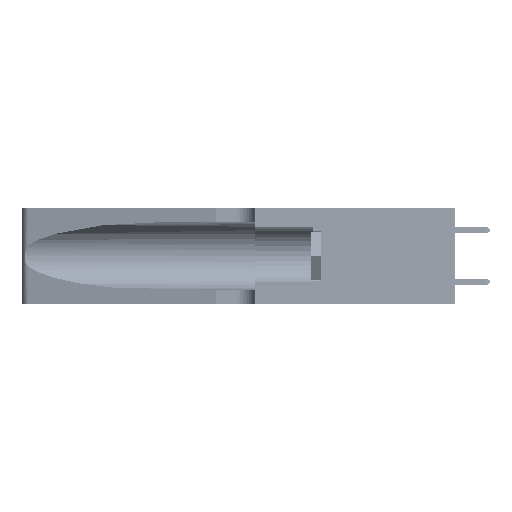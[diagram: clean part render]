
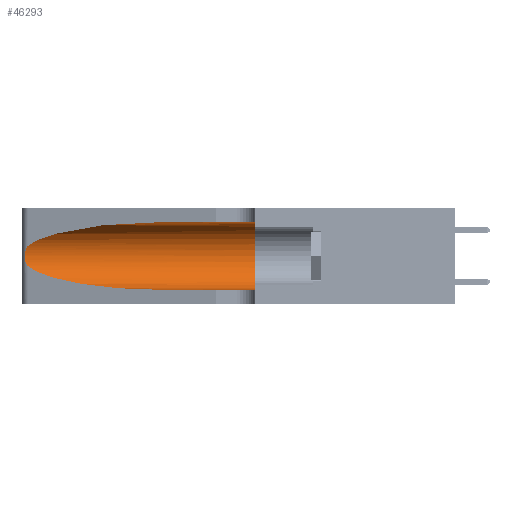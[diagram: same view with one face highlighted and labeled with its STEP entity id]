
A CAD part, left-side view. The second image highlights one B-rep face of the part: STEP entity #46293.
In plain terms, the highlighted cylindrical face has radius 3.308 mm (diameter 6.617 mm), a partial arc.
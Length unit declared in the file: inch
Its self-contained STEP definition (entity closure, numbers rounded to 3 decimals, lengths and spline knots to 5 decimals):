
#708 = EDGE_CURVE ( 'NONE', #19381, #9925, #44578, .T. ) ;
#1311 = LINE ( 'NONE', #46365, #7264 ) ;
#2916 = ORIENTED_EDGE ( 'NONE', *, *, #708, .T. ) ;
#4010 = VERTEX_POINT ( 'NONE', #32465 ) ;
#5555 = CARTESIAN_POINT ( 'NONE',  ( 0.2373, 1.15595, 0.28018 ) ) ;
#5770 = CARTESIAN_POINT ( 'NONE',  ( 0.25639, 1.23186, 0.15144 ) ) ;
#5934 = CARTESIAN_POINT ( 'NONE',  ( 0.25639, 1.23184, 0.21858 ) ) ;
#6511 = EDGE_CURVE ( 'NONE', #8257, #8683, #13293, .T. ) ;
#7264 = VECTOR ( 'NONE', #15856, 39.37008 ) ;
#8257 = VERTEX_POINT ( 'NONE', #29876 ) ;
#8683 = VERTEX_POINT ( 'NONE', #47180 ) ;
#8999 = B_SPLINE_CURVE_WITH_KNOTS ( 'NONE', 3,
 ( #17597, #44202, #5934, #24794, #32623, #44372, #21434, #24971, #24621, #9756, #21266, #5770, #29116, #20929 ),
 .UNSPECIFIED., .F., .F.,
 ( 4, 2, 2, 2, 2, 2, 4 ),
 ( 0., 0.00027, 0.00053, 0.00107, 0.0016, 0.00187, 0.00214 ),
 .UNSPECIFIED. ) ;
#9377 = CARTESIAN_POINT ( 'NONE',  ( 0.25487, 1.22718, 0.22369 ) ) ;
#9700 = CARTESIAN_POINT ( 'NONE',  ( 0.18966, 0.96281, 0.31525 ) ) ;
#9756 = CARTESIAN_POINT ( 'NONE',  ( 0.25856, 1.23593, 0.16098 ) ) ;
#9835 = CARTESIAN_POINT ( 'NONE',  ( 0.25487, 1.22718, 0.14631 ) ) ;
#9925 = VERTEX_POINT ( 'NONE', #40284 ) ;
#10850 = ORIENTED_EDGE ( 'NONE', *, *, #32089, .F. ) ;
#11664 = LINE ( 'NONE', #27835, #26010 ) ;
#13293 =( BOUNDED_CURVE ( )  B_SPLINE_CURVE ( 3, ( #35902, #9700, #5555, #9377 ),
 .UNSPECIFIED., .F., .T. ) 
 B_SPLINE_CURVE_WITH_KNOTS ( ( 4, 4 ),
 ( 1.5708, 2.84003 ),
 .UNSPECIFIED. ) 
 CURVE ( )  GEOMETRIC_REPRESENTATION_ITEM ( )  RATIONAL_B_SPLINE_CURVE ( ( 1., 0.87, 0.87, 1. ) ) 
 REPRESENTATION_ITEM ( '' )  );
#14222 = AXIS2_PLACEMENT_3D ( 'NONE', #48467, #25476, #21771 ) ;
#15856 = DIRECTION ( 'NONE',  ( 0., -1., 0. ) ) ;
#16618 = VERTEX_POINT ( 'NONE', #19991 ) ;
#17520 = CIRCLE ( 'NONE', #44090, 0.13025 ) ;
#17597 = CARTESIAN_POINT ( 'NONE',  ( 0.25487, 1.22718, 0.22369 ) ) ;
#19381 = VERTEX_POINT ( 'NONE', #45144 ) ;
#19991 = CARTESIAN_POINT ( 'NONE',  ( 0.1305, 0.35, 0.05475 ) ) ;
#20349 = ORIENTED_EDGE ( 'NONE', *, *, #31156, .F. ) ;
#20929 = CARTESIAN_POINT ( 'NONE',  ( 0.25487, 1.22718, 0.14631 ) ) ;
#21011 = CARTESIAN_POINT ( 'NONE',  ( 0.2373, 1.15595, 0.08982 ) ) ;
#21266 = CARTESIAN_POINT ( 'NONE',  ( 0.25789, 1.23486, 0.15765 ) ) ;
#21434 = CARTESIAN_POINT ( 'NONE',  ( 0.26075, 1.23896, 0.19203 ) ) ;
#21771 = DIRECTION ( 'NONE',  ( 0., 0., -1. ) ) ;
#21967 = EDGE_CURVE ( 'NONE', #9925, #16618, #11664, .T. ) ;
#24177 = DIRECTION ( 'NONE',  ( 0., -1., 0. ) ) ;
#24613 = EDGE_CURVE ( 'NONE', #8683, #19381, #8999, .T. ) ;
#24621 = CARTESIAN_POINT ( 'NONE',  ( 0.26017, 1.23833, 0.17102 ) ) ;
#24794 = CARTESIAN_POINT ( 'NONE',  ( 0.25787, 1.23484, 0.2124 ) ) ;
#24971 = CARTESIAN_POINT ( 'NONE',  ( 0.26075, 1.23896, 0.178 ) ) ;
#25476 = DIRECTION ( 'NONE',  ( 0., -1., 0. ) ) ;
#26010 = VECTOR ( 'NONE', #24177, 39.37008 ) ;
#27314 = CYLINDRICAL_SURFACE ( 'NONE', #14222, 0.13025 ) ;
#27835 = CARTESIAN_POINT ( 'NONE',  ( 0.1305, 1.61858, 0.05475 ) ) ;
#29116 = CARTESIAN_POINT ( 'NONE',  ( 0.25555, 1.22993, 0.14849 ) ) ;
#29876 = CARTESIAN_POINT ( 'NONE',  ( 0.1305, 0.72297, 0.31525 ) ) ;
#30116 = DIRECTION ( 'NONE',  ( 0., 1., 0. ) ) ;
#31156 = EDGE_CURVE ( 'NONE', #4010, #16618, #17520, .T. ) ;
#32089 = EDGE_CURVE ( 'NONE', #8257, #4010, #1311, .T. ) ;
#32371 = CARTESIAN_POINT ( 'NONE',  ( 0.18966, 0.96281, 0.05475 ) ) ;
#32465 = CARTESIAN_POINT ( 'NONE',  ( 0.1305, 0.35, 0.31525 ) ) ;
#32623 = CARTESIAN_POINT ( 'NONE',  ( 0.25854, 1.2359, 0.20912 ) ) ;
#34114 = DIRECTION ( 'NONE',  ( 0., 0., 1. ) ) ;
#35902 = CARTESIAN_POINT ( 'NONE',  ( 0.1305, 0.72297, 0.31525 ) ) ;
#37338 = ORIENTED_EDGE ( 'NONE', *, *, #6511, .T. ) ;
#37976 = CARTESIAN_POINT ( 'NONE',  ( 0.1305, 0.35, 0.185 ) ) ;
#39097 = ORIENTED_EDGE ( 'NONE', *, *, #24613, .T. ) ;
#40284 = CARTESIAN_POINT ( 'NONE',  ( 0.1305, 0.72297, 0.05475 ) ) ;
#42288 = FACE_OUTER_BOUND ( 'NONE', #43578, .T. ) ;
#43578 = EDGE_LOOP ( 'NONE', ( #37338, #39097, #2916, #45443, #20349, #10850 ) ) ;
#44090 = AXIS2_PLACEMENT_3D ( 'NONE', #37976, #30116, #34114 ) ;
#44202 = CARTESIAN_POINT ( 'NONE',  ( 0.25555, 1.22994, 0.2215 ) ) ;
#44372 = CARTESIAN_POINT ( 'NONE',  ( 0.26018, 1.23835, 0.19895 ) ) ;
#44578 =( BOUNDED_CURVE ( )  B_SPLINE_CURVE ( 3, ( #9835, #21011, #32371, #47549 ),
 .UNSPECIFIED., .F., .T. ) 
 B_SPLINE_CURVE_WITH_KNOTS ( ( 4, 4 ),
 ( 3.44316, 4.71239 ),
 .UNSPECIFIED. ) 
 CURVE ( )  GEOMETRIC_REPRESENTATION_ITEM ( )  RATIONAL_B_SPLINE_CURVE ( ( 1., 0.87, 0.87, 1. ) ) 
 REPRESENTATION_ITEM ( '' )  );
#45144 = CARTESIAN_POINT ( 'NONE',  ( 0.25487, 1.22718, 0.14631 ) ) ;
#45443 = ORIENTED_EDGE ( 'NONE', *, *, #21967, .T. ) ;
#46293 = ADVANCED_FACE ( 'NONE', ( #42288 ), #27314, .F. ) ;
#46365 = CARTESIAN_POINT ( 'NONE',  ( 0.1305, 1.61858, 0.31525 ) ) ;
#47180 = CARTESIAN_POINT ( 'NONE',  ( 0.25487, 1.22718, 0.22369 ) ) ;
#47549 = CARTESIAN_POINT ( 'NONE',  ( 0.1305, 0.72297, 0.05475 ) ) ;
#48467 = CARTESIAN_POINT ( 'NONE',  ( 0.1305, 1.61858, 0.185 ) ) ;
